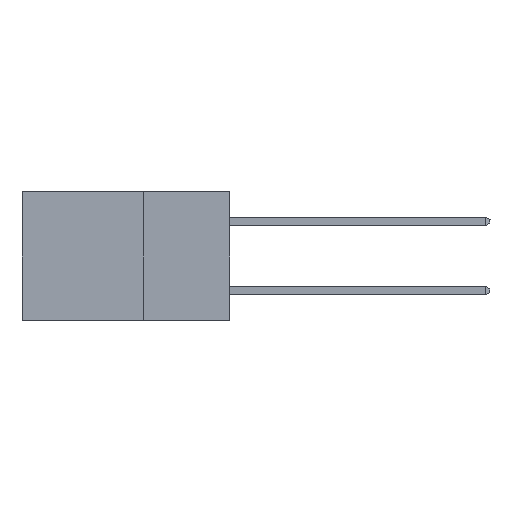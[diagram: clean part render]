
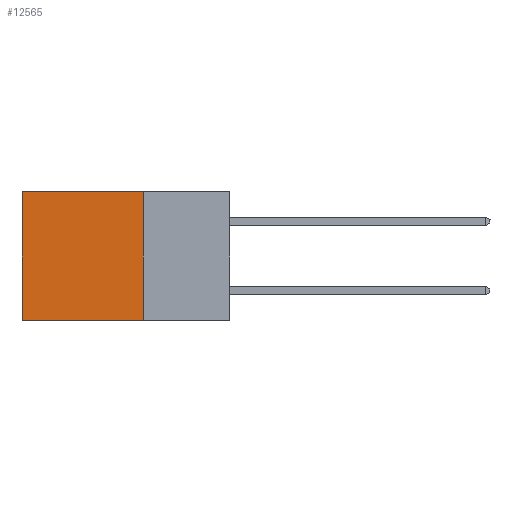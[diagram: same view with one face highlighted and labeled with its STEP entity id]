
A CAD part, left-side view. The second image highlights one B-rep face of the part: STEP entity #12565.
In plain terms, the highlighted planar face has unit normal (-1, 0, 0).
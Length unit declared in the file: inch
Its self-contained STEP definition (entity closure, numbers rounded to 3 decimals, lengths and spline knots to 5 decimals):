
#347 = EDGE_CURVE ( 'NONE', #12515, #13074, #1301, .T. ) ;
#1209 = DIRECTION ( 'NONE',  ( 0., 0., -1. ) ) ;
#1301 = LINE ( 'NONE', #5423, #7843 ) ;
#1398 = AXIS2_PLACEMENT_3D ( 'NONE', #15005, #7919, #8559 ) ;
#2337 = ORIENTED_EDGE ( 'NONE', *, *, #14075, .T. ) ;
#2761 = ORIENTED_EDGE ( 'NONE', *, *, #11557, .T. ) ;
#3797 = EDGE_LOOP ( 'NONE', ( #2761, #18171, #8678, #2337 ) ) ;
#5239 = CARTESIAN_POINT ( 'NONE',  ( 0.2615, 0.25, -0.37 ) ) ;
#5423 = CARTESIAN_POINT ( 'NONE',  ( 0.2615, 0.25, -0.37 ) ) ;
#6014 = VERTEX_POINT ( 'NONE', #11370 ) ;
#7843 = VECTOR ( 'NONE', #1209, 39.37008 ) ;
#7919 = DIRECTION ( 'NONE',  ( 1., 0., 0. ) ) ;
#8512 = DIRECTION ( 'NONE',  ( 0., 0., -1. ) ) ;
#8559 = DIRECTION ( 'NONE',  ( 0., 0., -1. ) ) ;
#8573 = VERTEX_POINT ( 'NONE', #16537 ) ;
#8678 = ORIENTED_EDGE ( 'NONE', *, *, #347, .F. ) ;
#9733 = CARTESIAN_POINT ( 'NONE',  ( 0.2615, 0.6, -0.37 ) ) ;
#9893 = VECTOR ( 'NONE', #8512, 39.37008 ) ;
#10713 = FACE_OUTER_BOUND ( 'NONE', #3797, .T. ) ;
#10966 = CARTESIAN_POINT ( 'NONE',  ( 0.2615, 0.25, -0.37 ) ) ;
#11370 = CARTESIAN_POINT ( 'NONE',  ( 0.2615, 0.6, 0. ) ) ;
#11557 = EDGE_CURVE ( 'NONE', #6014, #8573, #18321, .T. ) ;
#12027 = CARTESIAN_POINT ( 'NONE',  ( 0.2615, 0.25, 0. ) ) ;
#12418 = LINE ( 'NONE', #12511, #17275 ) ;
#12511 = CARTESIAN_POINT ( 'NONE',  ( 0.2615, 0.25, 0. ) ) ;
#12515 = VERTEX_POINT ( 'NONE', #12027 ) ;
#12534 = LINE ( 'NONE', #5239, #14282 ) ;
#12565 = ADVANCED_FACE ( 'NONE', ( #10713 ), #16390, .F. ) ;
#13074 = VERTEX_POINT ( 'NONE', #10966 ) ;
#14075 = EDGE_CURVE ( 'NONE', #12515, #6014, #12418, .T. ) ;
#14282 = VECTOR ( 'NONE', #15516, 39.37008 ) ;
#14818 = EDGE_CURVE ( 'NONE', #13074, #8573, #12534, .T. ) ;
#15005 = CARTESIAN_POINT ( 'NONE',  ( 0.2615, 0.25, -0.37 ) ) ;
#15308 = DIRECTION ( 'NONE',  ( 0., 1., 0. ) ) ;
#15516 = DIRECTION ( 'NONE',  ( 0., 1., 0. ) ) ;
#16390 = PLANE ( 'NONE',  #1398 ) ;
#16537 = CARTESIAN_POINT ( 'NONE',  ( 0.2615, 0.6, -0.37 ) ) ;
#17275 = VECTOR ( 'NONE', #15308, 39.37008 ) ;
#18171 = ORIENTED_EDGE ( 'NONE', *, *, #14818, .F. ) ;
#18321 = LINE ( 'NONE', #9733, #9893 ) ;
